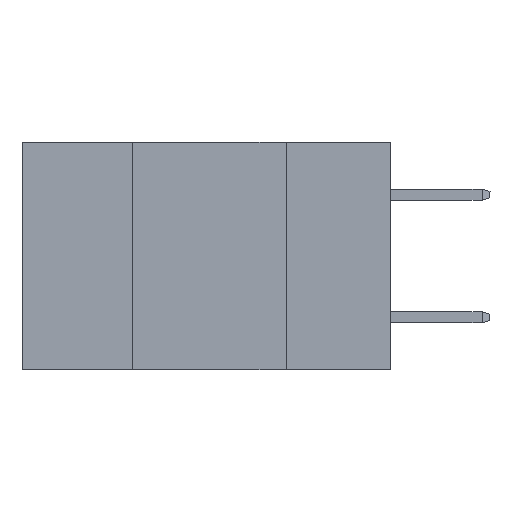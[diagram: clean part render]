
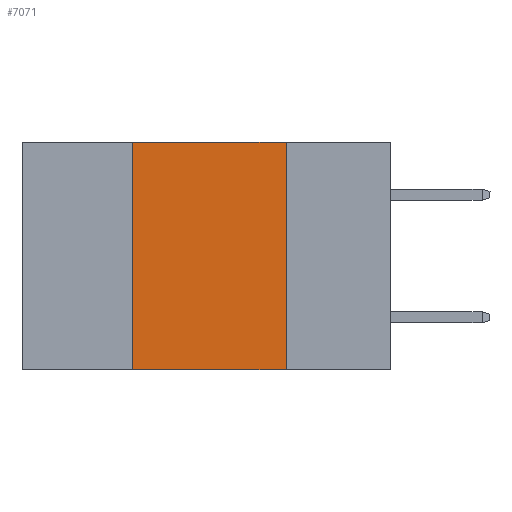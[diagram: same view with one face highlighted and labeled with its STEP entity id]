
A CAD part, left-side view. The second image highlights one B-rep face of the part: STEP entity #7071.
In plain terms, the highlighted planar face has unit normal (-1, 0, 0).
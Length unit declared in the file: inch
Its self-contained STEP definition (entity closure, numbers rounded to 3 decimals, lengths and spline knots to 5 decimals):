
#414 = ORIENTED_EDGE ( 'NONE', *, *, #9561, .F. ) ;
#545 = CARTESIAN_POINT ( 'NONE',  ( 0., 0.17, 0. ) ) ;
#551 = VECTOR ( 'NONE', #1223, 39.37008 ) ;
#757 = CARTESIAN_POINT ( 'NONE',  ( 0., 0.17, 0. ) ) ;
#1076 = EDGE_CURVE ( 'NONE', #3942, #1679, #6624, .T. ) ;
#1223 = DIRECTION ( 'NONE',  ( 0., 0., 1. ) ) ;
#1271 = ORIENTED_EDGE ( 'NONE', *, *, #5717, .F. ) ;
#1297 = CARTESIAN_POINT ( 'NONE',  ( 0., 0.17, -0.37 ) ) ;
#1679 = VERTEX_POINT ( 'NONE', #1962 ) ;
#1962 = CARTESIAN_POINT ( 'NONE',  ( 0., 0.42, 0. ) ) ;
#1971 = VECTOR ( 'NONE', #3126, 39.37008 ) ;
#2144 = FACE_OUTER_BOUND ( 'NONE', #2280, .T. ) ;
#2280 = EDGE_LOOP ( 'NONE', ( #414, #1271, #3624, #4553 ) ) ;
#3126 = DIRECTION ( 'NONE',  ( 0., 0., -1. ) ) ;
#3175 = CARTESIAN_POINT ( 'NONE',  ( 0., 0.6, 0. ) ) ;
#3247 = AXIS2_PLACEMENT_3D ( 'NONE', #3175, #9391, #4880 ) ;
#3277 = CARTESIAN_POINT ( 'NONE',  ( 0., 0.42, 0. ) ) ;
#3624 = ORIENTED_EDGE ( 'NONE', *, *, #1076, .F. ) ;
#3942 = VERTEX_POINT ( 'NONE', #7891 ) ;
#4229 = VERTEX_POINT ( 'NONE', #757 ) ;
#4484 = DIRECTION ( 'NONE',  ( 0., -1., 0. ) ) ;
#4553 = ORIENTED_EDGE ( 'NONE', *, *, #9259, .T. ) ;
#4880 = DIRECTION ( 'NONE',  ( 0., 0., -1. ) ) ;
#5717 = EDGE_CURVE ( 'NONE', #1679, #4229, #8033, .T. ) ;
#6008 = VECTOR ( 'NONE', #7919, 39.37008 ) ;
#6021 = CARTESIAN_POINT ( 'NONE',  ( 0., 0.6, -0.37 ) ) ;
#6624 = LINE ( 'NONE', #3277, #551 ) ;
#6769 = VECTOR ( 'NONE', #4484, 39.37008 ) ;
#7071 = ADVANCED_FACE ( 'NONE', ( #2144 ), #7933, .F. ) ;
#7636 = VERTEX_POINT ( 'NONE', #1297 ) ;
#7891 = CARTESIAN_POINT ( 'NONE',  ( 0., 0.42, -0.37 ) ) ;
#7919 = DIRECTION ( 'NONE',  ( 0., -1., 0. ) ) ;
#7933 = PLANE ( 'NONE',  #3247 ) ;
#8033 = LINE ( 'NONE', #9349, #6008 ) ;
#8544 = LINE ( 'NONE', #545, #1971 ) ;
#8754 = LINE ( 'NONE', #6021, #6769 ) ;
#9259 = EDGE_CURVE ( 'NONE', #3942, #7636, #8754, .T. ) ;
#9349 = CARTESIAN_POINT ( 'NONE',  ( 0., 0.6, 0. ) ) ;
#9391 = DIRECTION ( 'NONE',  ( 1., 0., 0. ) ) ;
#9561 = EDGE_CURVE ( 'NONE', #4229, #7636, #8544, .T. ) ;
